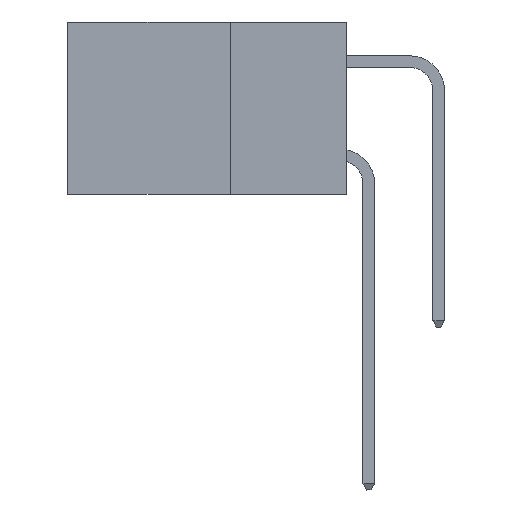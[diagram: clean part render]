
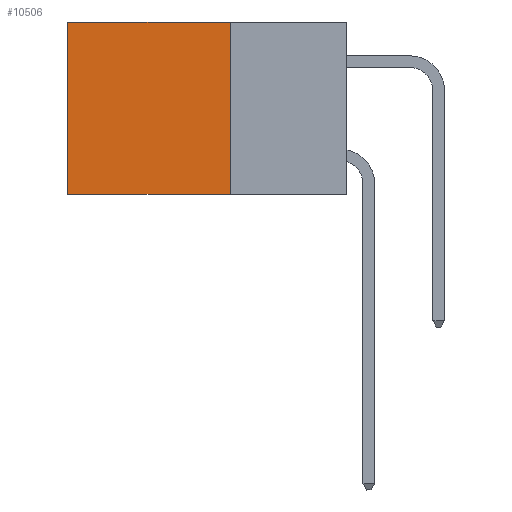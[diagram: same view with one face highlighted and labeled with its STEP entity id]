
A CAD part, left-side view. The second image highlights one B-rep face of the part: STEP entity #10506.
In plain terms, the highlighted planar face has unit normal (-1, 0, 0).
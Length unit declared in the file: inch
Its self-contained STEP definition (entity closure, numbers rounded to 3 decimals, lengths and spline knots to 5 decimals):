
#119 = EDGE_LOOP ( 'NONE', ( #23259, #9991, #13620, #24648 ) ) ;
#203 = CARTESIAN_POINT ( 'NONE',  ( 0.2875, 0.25, 0. ) ) ;
#347 = VERTEX_POINT ( 'NONE', #18563 ) ;
#830 = DIRECTION ( 'NONE',  ( 0., 0., -1. ) ) ;
#1752 = VERTEX_POINT ( 'NONE', #11358 ) ;
#2474 = DIRECTION ( 'NONE',  ( 0., 0., -1. ) ) ;
#2839 = CARTESIAN_POINT ( 'NONE',  ( 0.2875, 0.25, -0.37 ) ) ;
#3728 = EDGE_CURVE ( 'NONE', #347, #1752, #19909, .T. ) ;
#4623 = EDGE_CURVE ( 'NONE', #17573, #5935, #10659, .T. ) ;
#4772 = VECTOR ( 'NONE', #20893, 39.37008 ) ;
#5353 = AXIS2_PLACEMENT_3D ( 'NONE', #203, #6461, #2474 ) ;
#5696 = CARTESIAN_POINT ( 'NONE',  ( 0.2875, 0.25, 0. ) ) ;
#5935 = VERTEX_POINT ( 'NONE', #17043 ) ;
#5953 = VECTOR ( 'NONE', #13322, 39.37008 ) ;
#6461 = DIRECTION ( 'NONE',  ( 1., 0., 0. ) ) ;
#6731 = VECTOR ( 'NONE', #830, 39.37008 ) ;
#9507 = CARTESIAN_POINT ( 'NONE',  ( 0.2875, 0.6, 0. ) ) ;
#9991 = ORIENTED_EDGE ( 'NONE', *, *, #4623, .F. ) ;
#10327 = LINE ( 'NONE', #9507, #6731 ) ;
#10506 = ADVANCED_FACE ( 'NONE', ( #25918 ), #21655, .F. ) ;
#10659 = LINE ( 'NONE', #19501, #5953 ) ;
#11358 = CARTESIAN_POINT ( 'NONE',  ( 0.2875, 0.6, 0. ) ) ;
#11804 = EDGE_CURVE ( 'NONE', #347, #17573, #19330, .T. ) ;
#12513 = EDGE_CURVE ( 'NONE', #1752, #5935, #10327, .T. ) ;
#13322 = DIRECTION ( 'NONE',  ( 0., 1., 0. ) ) ;
#13620 = ORIENTED_EDGE ( 'NONE', *, *, #11804, .F. ) ;
#17043 = CARTESIAN_POINT ( 'NONE',  ( 0.2875, 0.6, -0.37 ) ) ;
#17573 = VERTEX_POINT ( 'NONE', #2839 ) ;
#18563 = CARTESIAN_POINT ( 'NONE',  ( 0.2875, 0.25, 0. ) ) ;
#19330 = LINE ( 'NONE', #5696, #4772 ) ;
#19501 = CARTESIAN_POINT ( 'NONE',  ( 0.2875, 0.25, -0.37 ) ) ;
#19909 = LINE ( 'NONE', #20034, #25708 ) ;
#20034 = CARTESIAN_POINT ( 'NONE',  ( 0.2875, 0.25, 0. ) ) ;
#20893 = DIRECTION ( 'NONE',  ( 0., 0., -1. ) ) ;
#21655 = PLANE ( 'NONE',  #5353 ) ;
#23259 = ORIENTED_EDGE ( 'NONE', *, *, #12513, .T. ) ;
#24648 = ORIENTED_EDGE ( 'NONE', *, *, #3728, .T. ) ;
#25708 = VECTOR ( 'NONE', #26631, 39.37008 ) ;
#25918 = FACE_OUTER_BOUND ( 'NONE', #119, .T. ) ;
#26631 = DIRECTION ( 'NONE',  ( 0., 1., 0. ) ) ;
